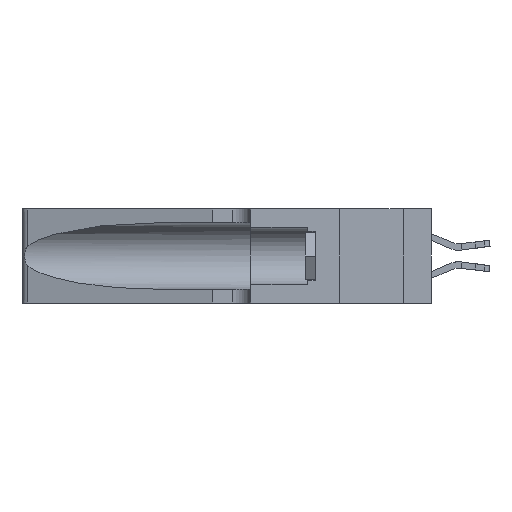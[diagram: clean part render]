
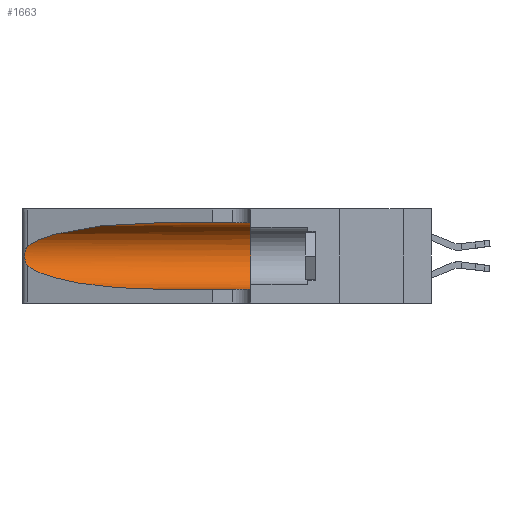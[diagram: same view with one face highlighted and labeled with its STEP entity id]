
A CAD part, left-side view. The second image highlights one B-rep face of the part: STEP entity #1663.
In plain terms, the highlighted cylindrical face has radius 3.308 mm (diameter 6.617 mm), a partial arc.
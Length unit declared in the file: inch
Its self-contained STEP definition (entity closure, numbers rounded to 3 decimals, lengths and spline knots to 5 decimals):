
#83 = CARTESIAN_POINT ( 'NONE',  ( 0.25555, 1.22994, 0.2215 ) ) ;
#486 = VERTEX_POINT ( 'NONE', #12926 ) ;
#1663 = ADVANCED_FACE ( 'NONE', ( #15789 ), #8108, .F. ) ;
#2262 = DIRECTION ( 'NONE',  ( 0., -1., 0. ) ) ;
#2301 = VERTEX_POINT ( 'NONE', #15438 ) ;
#2358 = CARTESIAN_POINT ( 'NONE',  ( 0.25487, 1.22718, 0.14631 ) ) ;
#2740 = AXIS2_PLACEMENT_3D ( 'NONE', #14573, #7839, #17810 ) ;
#3177 = CARTESIAN_POINT ( 'NONE',  ( 0.25854, 1.2359, 0.20912 ) ) ;
#3489 = CARTESIAN_POINT ( 'NONE',  ( 0.25487, 1.22718, 0.22369 ) ) ;
#3971 = DIRECTION ( 'NONE',  ( 0., 0., -1. ) ) ;
#4063 = CARTESIAN_POINT ( 'NONE',  ( 0.2373, 1.15595, 0.08982 ) ) ;
#4220 = EDGE_CURVE ( 'NONE', #2301, #486, #4822, .T. ) ;
#4822 = LINE ( 'NONE', #15462, #15934 ) ;
#4862 = CARTESIAN_POINT ( 'NONE',  ( 0.26017, 1.23833, 0.17102 ) ) ;
#5005 = CARTESIAN_POINT ( 'NONE',  ( 0.25856, 1.23593, 0.16098 ) ) ;
#5554 = VERTEX_POINT ( 'NONE', #14111 ) ;
#6729 = VERTEX_POINT ( 'NONE', #17729 ) ;
#7289 = CARTESIAN_POINT ( 'NONE',  ( 0.1305, 1.61858, 0.185 ) ) ;
#7418 = EDGE_CURVE ( 'NONE', #5554, #7911, #21637, .T. ) ;
#7839 = DIRECTION ( 'NONE',  ( 0., 1., 0. ) ) ;
#7911 = VERTEX_POINT ( 'NONE', #16734 ) ;
#8108 = CYLINDRICAL_SURFACE ( 'NONE', #14079, 0.13025 ) ;
#8321 = CARTESIAN_POINT ( 'NONE',  ( 0.25787, 1.23484, 0.2124 ) ) ;
#8449 = EDGE_LOOP ( 'NONE', ( #9589, #14997, #10122, #18163, #11053, #14830 ) ) ;
#9589 = ORIENTED_EDGE ( 'NONE', *, *, #12502, .T. ) ;
#10096 = CARTESIAN_POINT ( 'NONE',  ( 0.25555, 1.22993, 0.14849 ) ) ;
#10122 = ORIENTED_EDGE ( 'NONE', *, *, #13255, .T. ) ;
#11053 = ORIENTED_EDGE ( 'NONE', *, *, #11967, .F. ) ;
#11659 = CARTESIAN_POINT ( 'NONE',  ( 0.25639, 1.23184, 0.21858 ) ) ;
#11807 = CARTESIAN_POINT ( 'NONE',  ( 0.26075, 1.23896, 0.178 ) ) ;
#11967 = EDGE_CURVE ( 'NONE', #6729, #486, #18134, .T. ) ;
#12349 = VERTEX_POINT ( 'NONE', #17561 ) ;
#12443 = DIRECTION ( 'NONE',  ( 0., -1., 0. ) ) ;
#12502 = EDGE_CURVE ( 'NONE', #12349, #5554, #21234, .T. ) ;
#12926 = CARTESIAN_POINT ( 'NONE',  ( 0.1305, 0.35, 0.05475 ) ) ;
#13255 = EDGE_CURVE ( 'NONE', #7911, #2301, #20546, .T. ) ;
#13905 = EDGE_CURVE ( 'NONE', #12349, #6729, #15606, .T. ) ;
#14079 = AXIS2_PLACEMENT_3D ( 'NONE', #7289, #2262, #3971 ) ;
#14111 = CARTESIAN_POINT ( 'NONE',  ( 0.25487, 1.22718, 0.22369 ) ) ;
#14573 = CARTESIAN_POINT ( 'NONE',  ( 0.1305, 0.35, 0.185 ) ) ;
#14830 = ORIENTED_EDGE ( 'NONE', *, *, #13905, .F. ) ;
#14997 = ORIENTED_EDGE ( 'NONE', *, *, #7418, .T. ) ;
#15069 = CARTESIAN_POINT ( 'NONE',  ( 0.26018, 1.23835, 0.19895 ) ) ;
#15100 = CARTESIAN_POINT ( 'NONE',  ( 0.2373, 1.15595, 0.28018 ) ) ;
#15438 = CARTESIAN_POINT ( 'NONE',  ( 0.1305, 0.72297, 0.05475 ) ) ;
#15462 = CARTESIAN_POINT ( 'NONE',  ( 0.1305, 1.61858, 0.05475 ) ) ;
#15606 = LINE ( 'NONE', #21944, #17464 ) ;
#15789 = FACE_OUTER_BOUND ( 'NONE', #8449, .T. ) ;
#15934 = VECTOR ( 'NONE', #17165, 39.37008 ) ;
#16734 = CARTESIAN_POINT ( 'NONE',  ( 0.25487, 1.22718, 0.14631 ) ) ;
#16778 = CARTESIAN_POINT ( 'NONE',  ( 0.25639, 1.23186, 0.15144 ) ) ;
#17165 = DIRECTION ( 'NONE',  ( 0., -1., 0. ) ) ;
#17300 = CARTESIAN_POINT ( 'NONE',  ( 0.18966, 0.96281, 0.05475 ) ) ;
#17380 = CARTESIAN_POINT ( 'NONE',  ( 0.1305, 0.72297, 0.05475 ) ) ;
#17464 = VECTOR ( 'NONE', #12443, 39.37008 ) ;
#17561 = CARTESIAN_POINT ( 'NONE',  ( 0.1305, 0.72297, 0.31525 ) ) ;
#17729 = CARTESIAN_POINT ( 'NONE',  ( 0.1305, 0.35, 0.31525 ) ) ;
#17810 = DIRECTION ( 'NONE',  ( 0., 0., 1. ) ) ;
#17987 = CARTESIAN_POINT ( 'NONE',  ( 0.1305, 0.72297, 0.31525 ) ) ;
#18134 = CIRCLE ( 'NONE', #2740, 0.13025 ) ;
#18163 = ORIENTED_EDGE ( 'NONE', *, *, #4220, .T. ) ;
#18404 = CARTESIAN_POINT ( 'NONE',  ( 0.26075, 1.23896, 0.19203 ) ) ;
#18549 = CARTESIAN_POINT ( 'NONE',  ( 0.25487, 1.22718, 0.14631 ) ) ;
#19645 = CARTESIAN_POINT ( 'NONE',  ( 0.25789, 1.23486, 0.15765 ) ) ;
#19791 = CARTESIAN_POINT ( 'NONE',  ( 0.18966, 0.96281, 0.31525 ) ) ;
#20546 =( BOUNDED_CURVE ( )  B_SPLINE_CURVE ( 3, ( #2358, #4063, #17300, #17380 ),
 .UNSPECIFIED., .F., .T. ) 
 B_SPLINE_CURVE_WITH_KNOTS ( ( 4, 4 ),
 ( 3.44316, 4.71239 ),
 .UNSPECIFIED. ) 
 CURVE ( )  GEOMETRIC_REPRESENTATION_ITEM ( )  RATIONAL_B_SPLINE_CURVE ( ( 1., 0.87, 0.87, 1. ) ) 
 REPRESENTATION_ITEM ( '' )  );
#21234 =( BOUNDED_CURVE ( )  B_SPLINE_CURVE ( 3, ( #17987, #19791, #15100, #3489 ),
 .UNSPECIFIED., .F., .F. ) 
 B_SPLINE_CURVE_WITH_KNOTS ( ( 4, 4 ),
 ( 1.5708, 2.84003 ),
 .UNSPECIFIED. ) 
 CURVE ( )  GEOMETRIC_REPRESENTATION_ITEM ( )  RATIONAL_B_SPLINE_CURVE ( ( 1., 0.87, 0.87, 1. ) ) 
 REPRESENTATION_ITEM ( '' )  );
#21637 = B_SPLINE_CURVE_WITH_KNOTS ( 'NONE', 3,
 ( #21878, #83, #11659, #8321, #3177, #15069, #18404, #11807, #4862, #5005, #19645, #16778, #10096, #18549 ),
 .UNSPECIFIED., .F., .F.,
 ( 4, 2, 2, 2, 2, 2, 4 ),
 ( 0., 0.00027, 0.00053, 0.00107, 0.0016, 0.00187, 0.00214 ),
 .UNSPECIFIED. ) ;
#21878 = CARTESIAN_POINT ( 'NONE',  ( 0.25487, 1.22718, 0.22369 ) ) ;
#21944 = CARTESIAN_POINT ( 'NONE',  ( 0.1305, 1.61858, 0.31525 ) ) ;
